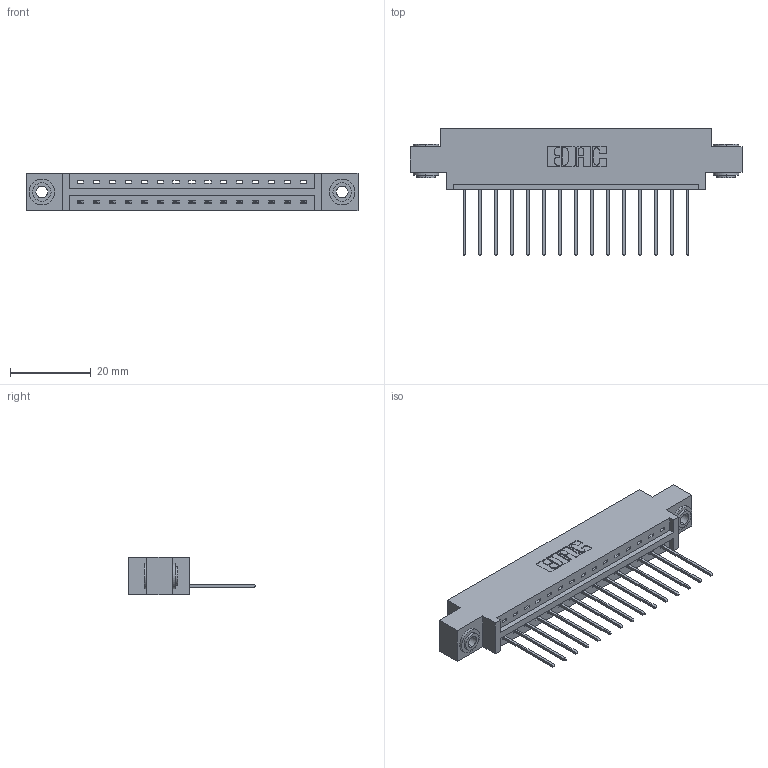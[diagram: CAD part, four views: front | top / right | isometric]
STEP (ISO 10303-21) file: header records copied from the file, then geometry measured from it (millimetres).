
FILE_DESCRIPTION (( 'STEP AP203' ), '1' );
FILE_NAME ('387-015-542-603.STEP', '2019-10-02T17:42:17', ( '' ), ( '' ), 'SwSTEP 2.0', 'SolidWorks 2016', '' );
FILE_SCHEMA (( 'CONFIG_CONTROL_DESIGN' ));
Length unit declared in the file: inch
Products named in the file (4): 337 Part_0.170 Offset - 0.156 Dia-TH; 345-292-001_345-293-142; 387-015-542-603; 345-250-002_345-250-002-102
Assembly tree (18 placements, depth 2):
  387-015-542-603
    337 Part_0.170 Offset - 0.156 Dia-TH
    345-292-001_345-293-142  x15
    345-250-002_345-250-002-102  x2
Bounding box: 82.45 x 31.63 x 9.4 mm (x, y, z)
Volume: 8166.5 mm3; surface area: 8837.7 mm2
Topology: 18 solids, 18 shells, 1086 faces, 3219 edges, 2122 vertices
Faces by surface type: plane 774, cylinder 304, cone 8
Entity records: 15442 total; most frequent: CARTESIAN_POINT 2666, ORIENTED_EDGE 2610, DIRECTION 2333, EDGE_CURVE 1305, VECTOR 1153, LINE 1153, VERTEX_POINT 866, AXIS2_PLACEMENT_3D 590
